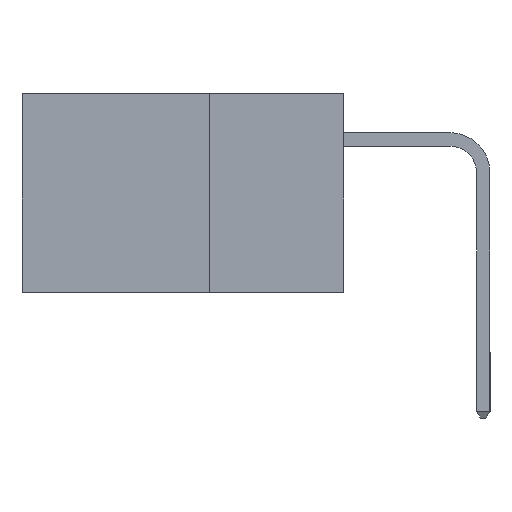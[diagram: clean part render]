
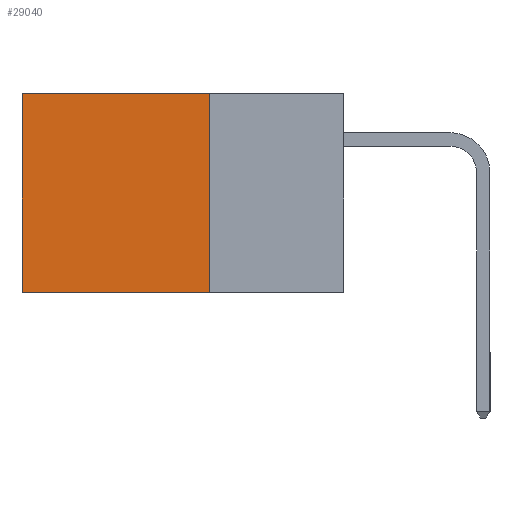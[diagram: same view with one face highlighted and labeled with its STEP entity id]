
A CAD part, left-side view. The second image highlights one B-rep face of the part: STEP entity #29040.
In plain terms, the highlighted planar face has unit normal (-1, 0, 0).
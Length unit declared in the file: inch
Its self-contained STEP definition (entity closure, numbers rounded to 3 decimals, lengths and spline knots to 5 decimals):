
#1143 = CARTESIAN_POINT ( 'NONE',  ( 0.298, 0.25, -0.37 ) ) ;
#1255 = CARTESIAN_POINT ( 'NONE',  ( 0.298, 0.25, 0. ) ) ;
#2067 = VERTEX_POINT ( 'NONE', #8667 ) ;
#2079 = DIRECTION ( 'NONE',  ( 0., 0., -1. ) ) ;
#2710 = CARTESIAN_POINT ( 'NONE',  ( 0.298, 0.25, 0. ) ) ;
#3358 = CARTESIAN_POINT ( 'NONE',  ( 0.298, 0.25, 0. ) ) ;
#5227 = VERTEX_POINT ( 'NONE', #5779 ) ;
#5779 = CARTESIAN_POINT ( 'NONE',  ( 0.298, 0.25, -0.37 ) ) ;
#5942 = DIRECTION ( 'NONE',  ( 1., 0., 0. ) ) ;
#6885 = LINE ( 'NONE', #1255, #32465 ) ;
#7401 = EDGE_CURVE ( 'NONE', #2067, #8216, #16893, .T. ) ;
#8216 = VERTEX_POINT ( 'NONE', #31793 ) ;
#8667 = CARTESIAN_POINT ( 'NONE',  ( 0.298, 0.25, 0. ) ) ;
#11781 = FACE_OUTER_BOUND ( 'NONE', #16626, .T. ) ;
#13300 = EDGE_CURVE ( 'NONE', #8216, #14963, #21459, .T. ) ;
#13847 = VECTOR ( 'NONE', #2079, 39.37008 ) ;
#14059 = ORIENTED_EDGE ( 'NONE', *, *, #7401, .T. ) ;
#14589 = ORIENTED_EDGE ( 'NONE', *, *, #14991, .F. ) ;
#14963 = VERTEX_POINT ( 'NONE', #29089 ) ;
#14991 = EDGE_CURVE ( 'NONE', #2067, #5227, #6885, .T. ) ;
#16611 = DIRECTION ( 'NONE',  ( 0., 0., -1. ) ) ;
#16626 = EDGE_LOOP ( 'NONE', ( #18985, #26419, #14589, #14059 ) ) ;
#16800 = EDGE_CURVE ( 'NONE', #5227, #14963, #22768, .T. ) ;
#16893 = LINE ( 'NONE', #2710, #29636 ) ;
#17595 = VECTOR ( 'NONE', #19079, 39.37008 ) ;
#17596 = AXIS2_PLACEMENT_3D ( 'NONE', #3358, #5942, #23829 ) ;
#18077 = DIRECTION ( 'NONE',  ( 0., 1., 0. ) ) ;
#18728 = PLANE ( 'NONE',  #17596 ) ;
#18985 = ORIENTED_EDGE ( 'NONE', *, *, #13300, .T. ) ;
#19079 = DIRECTION ( 'NONE',  ( 0., 1., 0. ) ) ;
#20005 = CARTESIAN_POINT ( 'NONE',  ( 0.298, 0.6, 0. ) ) ;
#21459 = LINE ( 'NONE', #20005, #13847 ) ;
#22768 = LINE ( 'NONE', #1143, #17595 ) ;
#23829 = DIRECTION ( 'NONE',  ( 0., 0., -1. ) ) ;
#26419 = ORIENTED_EDGE ( 'NONE', *, *, #16800, .F. ) ;
#29040 = ADVANCED_FACE ( 'NONE', ( #11781 ), #18728, .F. ) ;
#29089 = CARTESIAN_POINT ( 'NONE',  ( 0.298, 0.6, -0.37 ) ) ;
#29636 = VECTOR ( 'NONE', #18077, 39.37008 ) ;
#31793 = CARTESIAN_POINT ( 'NONE',  ( 0.298, 0.6, 0. ) ) ;
#32465 = VECTOR ( 'NONE', #16611, 39.37008 ) ;
